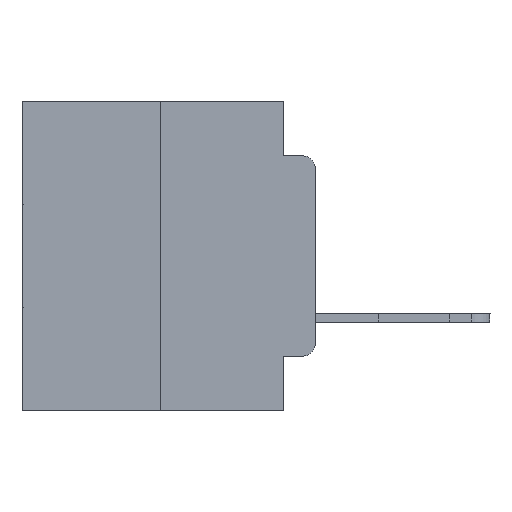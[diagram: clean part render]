
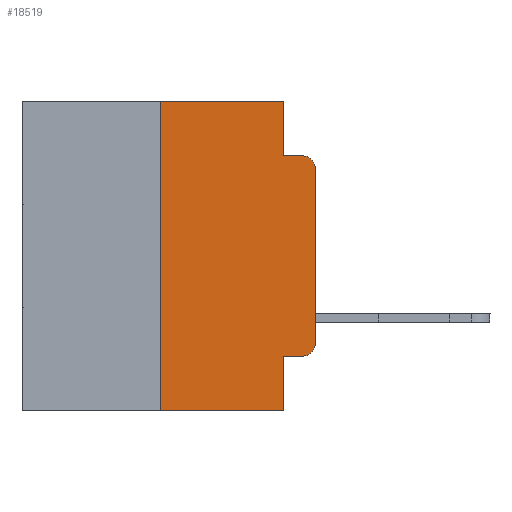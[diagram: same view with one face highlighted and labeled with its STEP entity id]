
A CAD part, left-side view. The second image highlights one B-rep face of the part: STEP entity #18519.
In plain terms, the highlighted planar face has unit normal (-1, 0, 0).
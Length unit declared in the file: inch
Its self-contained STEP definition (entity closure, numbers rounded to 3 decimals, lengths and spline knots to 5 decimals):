
#649 = VERTEX_POINT ( 'NONE', #11213 ) ;
#746 = CARTESIAN_POINT ( 'NONE',  ( 0., 0.051, -0.4115 ) ) ;
#792 = ORIENTED_EDGE ( 'NONE', *, *, #25766, .F. ) ;
#1224 = DIRECTION ( 'NONE',  ( 1., 0., 0. ) ) ;
#2067 = DIRECTION ( 'NONE',  ( -1., 0., 0. ) ) ;
#2369 = ORIENTED_EDGE ( 'NONE', *, *, #12208, .F. ) ;
#2447 = DIRECTION ( 'NONE',  ( 0., 0., -1. ) ) ;
#2608 = CARTESIAN_POINT ( 'NONE',  ( 0., 0.473, 0. ) ) ;
#4413 = LINE ( 'NONE', #6064, #6715 ) ;
#4903 = EDGE_CURVE ( 'NONE', #13414, #20784, #15440, .T. ) ;
#4919 = CARTESIAN_POINT ( 'NONE',  ( 0., 0.051, 0. ) ) ;
#5379 = ORIENTED_EDGE ( 'NONE', *, *, #4903, .T. ) ;
#5631 = AXIS2_PLACEMENT_3D ( 'NONE', #19809, #1224, #7610 ) ;
#5660 = LINE ( 'NONE', #26300, #25923 ) ;
#5788 = DIRECTION ( 'NONE',  ( 0., -1., 0. ) ) ;
#6008 = DIRECTION ( 'NONE',  ( 0., 0., 1. ) ) ;
#6064 = CARTESIAN_POINT ( 'NONE',  ( 0., 0., 0. ) ) ;
#6639 = CIRCLE ( 'NONE', #10096, 0.02 ) ;
#6715 = VECTOR ( 'NONE', #14320, 39.37008 ) ;
#7184 = CARTESIAN_POINT ( 'NONE',  ( 0., 0.051, 0. ) ) ;
#7202 = EDGE_CURVE ( 'NONE', #8514, #19325, #5660, .T. ) ;
#7243 = VERTEX_POINT ( 'NONE', #26834 ) ;
#7610 = DIRECTION ( 'NONE',  ( 0., 0., -1. ) ) ;
#7880 = EDGE_CURVE ( 'NONE', #8514, #7243, #23621, .T. ) ;
#8226 = VECTOR ( 'NONE', #25100, 39.37008 ) ;
#8426 = CARTESIAN_POINT ( 'NONE',  ( 0., 0.473, -0.5 ) ) ;
#8514 = VERTEX_POINT ( 'NONE', #746 ) ;
#9209 = LINE ( 'NONE', #7184, #13676 ) ;
#9644 = VERTEX_POINT ( 'NONE', #13964 ) ;
#9777 = ORIENTED_EDGE ( 'NONE', *, *, #12262, .T. ) ;
#10096 = AXIS2_PLACEMENT_3D ( 'NONE', #25396, #10742, #2447 ) ;
#10194 = LINE ( 'NONE', #14522, #20513 ) ;
#10313 = EDGE_CURVE ( 'NONE', #9644, #24831, #21228, .T. ) ;
#10742 = DIRECTION ( 'NONE',  ( -1., 0., 0. ) ) ;
#10893 = DIRECTION ( 'NONE',  ( 0., -1., 0. ) ) ;
#10992 = DIRECTION ( 'NONE',  ( 0., -1., 0. ) ) ;
#11056 = EDGE_CURVE ( 'NONE', #24826, #20784, #21197, .T. ) ;
#11213 = CARTESIAN_POINT ( 'NONE',  ( 0., 0.25, -0.5 ) ) ;
#11375 = DIRECTION ( 'NONE',  ( 0., 0., -1. ) ) ;
#11916 = DIRECTION ( 'NONE',  ( 0., 0., -1. ) ) ;
#12208 = EDGE_CURVE ( 'NONE', #649, #9644, #10194, .T. ) ;
#12262 = EDGE_CURVE ( 'NONE', #19325, #25569, #6639, .T. ) ;
#12617 = VECTOR ( 'NONE', #11916, 39.37008 ) ;
#12854 = CARTESIAN_POINT ( 'NONE',  ( 0., 0., -0.3915 ) ) ;
#13371 = CARTESIAN_POINT ( 'NONE',  ( 0., 0.051, 0. ) ) ;
#13414 = VERTEX_POINT ( 'NONE', #20154 ) ;
#13676 = VECTOR ( 'NONE', #11375, 39.37008 ) ;
#13964 = CARTESIAN_POINT ( 'NONE',  ( 0., 0.25, 0. ) ) ;
#14135 = CARTESIAN_POINT ( 'NONE',  ( 0., 0.02, -0.4115 ) ) ;
#14310 = CARTESIAN_POINT ( 'NONE',  ( 0., 0.02, -0.0885 ) ) ;
#14320 = DIRECTION ( 'NONE',  ( 0., 0., 1. ) ) ;
#14501 = LINE ( 'NONE', #8426, #8226 ) ;
#14522 = CARTESIAN_POINT ( 'NONE',  ( 0., 0.25, 0. ) ) ;
#15440 = CIRCLE ( 'NONE', #17671, 0.02 ) ;
#16713 = DIRECTION ( 'NONE',  ( 0., 0., -1. ) ) ;
#17671 = AXIS2_PLACEMENT_3D ( 'NONE', #26806, #2067, #16713 ) ;
#17718 = VECTOR ( 'NONE', #10893, 39.37008 ) ;
#17871 = ORIENTED_EDGE ( 'NONE', *, *, #7880, .F. ) ;
#18189 = ORIENTED_EDGE ( 'NONE', *, *, #20002, .T. ) ;
#18519 = ADVANCED_FACE ( 'NONE', ( #26074 ), #26204, .F. ) ;
#19325 = VERTEX_POINT ( 'NONE', #14135 ) ;
#19809 = CARTESIAN_POINT ( 'NONE',  ( 0., 0.473, 0. ) ) ;
#20002 = EDGE_CURVE ( 'NONE', #649, #7243, #14501, .T. ) ;
#20154 = CARTESIAN_POINT ( 'NONE',  ( 0., 0., -0.1085 ) ) ;
#20513 = VECTOR ( 'NONE', #6008, 39.37008 ) ;
#20623 = ORIENTED_EDGE ( 'NONE', *, *, #24777, .T. ) ;
#20784 = VERTEX_POINT ( 'NONE', #14310 ) ;
#21197 = LINE ( 'NONE', #21330, #26341 ) ;
#21228 = LINE ( 'NONE', #2608, #17718 ) ;
#21330 = CARTESIAN_POINT ( 'NONE',  ( 0., 0.051, -0.0885 ) ) ;
#21681 = ORIENTED_EDGE ( 'NONE', *, *, #7202, .T. ) ;
#22496 = ORIENTED_EDGE ( 'NONE', *, *, #10313, .F. ) ;
#23621 = LINE ( 'NONE', #4919, #12617 ) ;
#23673 = CARTESIAN_POINT ( 'NONE',  ( 0., 0.051, -0.0885 ) ) ;
#24777 = EDGE_CURVE ( 'NONE', #25569, #13414, #4413, .T. ) ;
#24826 = VERTEX_POINT ( 'NONE', #23673 ) ;
#24831 = VERTEX_POINT ( 'NONE', #13371 ) ;
#24865 = EDGE_LOOP ( 'NONE', ( #20623, #5379, #25419, #792, #22496, #2369, #18189, #17871, #21681, #9777 ) ) ;
#25100 = DIRECTION ( 'NONE',  ( 0., -1., 0. ) ) ;
#25396 = CARTESIAN_POINT ( 'NONE',  ( 0., 0.02, -0.3915 ) ) ;
#25419 = ORIENTED_EDGE ( 'NONE', *, *, #11056, .F. ) ;
#25569 = VERTEX_POINT ( 'NONE', #12854 ) ;
#25766 = EDGE_CURVE ( 'NONE', #24831, #24826, #9209, .T. ) ;
#25923 = VECTOR ( 'NONE', #5788, 39.37008 ) ;
#26074 = FACE_OUTER_BOUND ( 'NONE', #24865, .T. ) ;
#26204 = PLANE ( 'NONE',  #5631 ) ;
#26300 = CARTESIAN_POINT ( 'NONE',  ( 0., 0.051, -0.4115 ) ) ;
#26341 = VECTOR ( 'NONE', #10992, 39.37008 ) ;
#26806 = CARTESIAN_POINT ( 'NONE',  ( 0., 0.02, -0.1085 ) ) ;
#26834 = CARTESIAN_POINT ( 'NONE',  ( 0., 0.051, -0.5 ) ) ;
